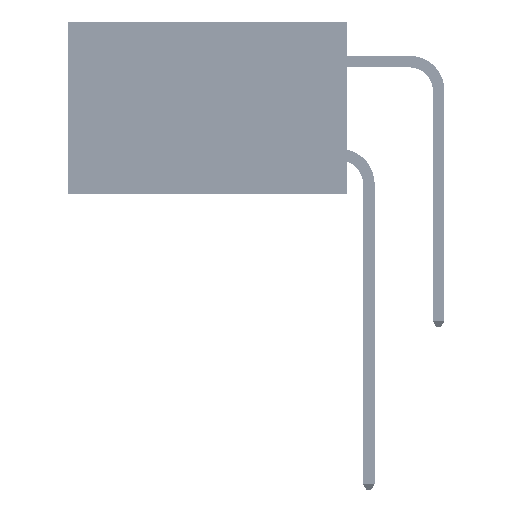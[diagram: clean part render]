
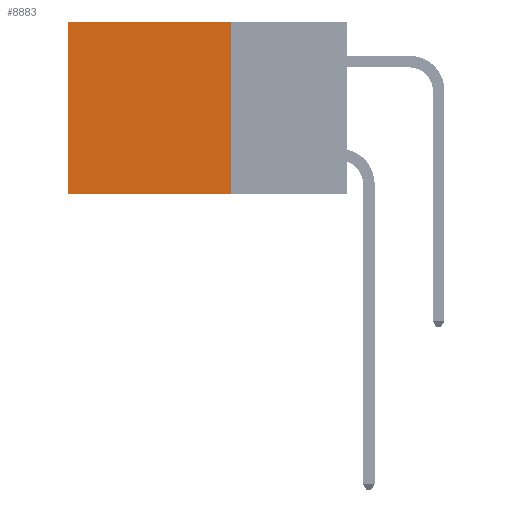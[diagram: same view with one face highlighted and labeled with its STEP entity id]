
A CAD part, left-side view. The second image highlights one B-rep face of the part: STEP entity #8883.
In plain terms, the highlighted planar face has unit normal (-1, 0, 0).
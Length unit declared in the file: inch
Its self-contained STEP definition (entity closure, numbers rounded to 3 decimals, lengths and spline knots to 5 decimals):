
#1233 = CARTESIAN_POINT ( 'NONE',  ( 0.2875, 0.25, 0. ) ) ;
#2089 = CARTESIAN_POINT ( 'NONE',  ( 0.2875, 0.25, -0.37 ) ) ;
#4699 = ORIENTED_EDGE ( 'NONE', *, *, #13519, .F. ) ;
#6615 = LINE ( 'NONE', #29673, #27354 ) ;
#8883 = ADVANCED_FACE ( 'NONE', ( #36243 ), #31109, .F. ) ;
#9104 = DIRECTION ( 'NONE',  ( 0., 1., 0. ) ) ;
#9928 = VERTEX_POINT ( 'NONE', #2089 ) ;
#10130 = VECTOR ( 'NONE', #17261, 39.37008 ) ;
#13519 = EDGE_CURVE ( 'NONE', #16123, #9928, #17411, .T. ) ;
#13660 = CARTESIAN_POINT ( 'NONE',  ( 0.2875, 0.25, 0. ) ) ;
#15400 = ORIENTED_EDGE ( 'NONE', *, *, #16861, .F. ) ;
#16123 = VERTEX_POINT ( 'NONE', #1233 ) ;
#16579 = CARTESIAN_POINT ( 'NONE',  ( 0.2875, 0.25, 0. ) ) ;
#16861 = EDGE_CURVE ( 'NONE', #9928, #22538, #6615, .T. ) ;
#17261 = DIRECTION ( 'NONE',  ( 0., 0., -1. ) ) ;
#17411 = LINE ( 'NONE', #13660, #10130 ) ;
#19578 = LINE ( 'NONE', #30845, #31852 ) ;
#20511 = DIRECTION ( 'NONE',  ( 1., 0., 0. ) ) ;
#20613 = ORIENTED_EDGE ( 'NONE', *, *, #42983, .T. ) ;
#22538 = VERTEX_POINT ( 'NONE', #30517 ) ;
#25399 = EDGE_LOOP ( 'NONE', ( #20613, #15400, #4699, #40472 ) ) ;
#27354 = VECTOR ( 'NONE', #44511, 39.37008 ) ;
#27930 = AXIS2_PLACEMENT_3D ( 'NONE', #16579, #20511, #45489 ) ;
#29030 = CARTESIAN_POINT ( 'NONE',  ( 0.2875, 0.6, 0. ) ) ;
#29673 = CARTESIAN_POINT ( 'NONE',  ( 0.2875, 0.25, -0.37 ) ) ;
#30293 = EDGE_CURVE ( 'NONE', #16123, #36213, #19578, .T. ) ;
#30517 = CARTESIAN_POINT ( 'NONE',  ( 0.2875, 0.6, -0.37 ) ) ;
#30731 = VECTOR ( 'NONE', #32279, 39.37008 ) ;
#30845 = CARTESIAN_POINT ( 'NONE',  ( 0.2875, 0.25, 0. ) ) ;
#31109 = PLANE ( 'NONE',  #27930 ) ;
#31852 = VECTOR ( 'NONE', #9104, 39.37008 ) ;
#32279 = DIRECTION ( 'NONE',  ( 0., 0., -1. ) ) ;
#33496 = LINE ( 'NONE', #44782, #30731 ) ;
#36213 = VERTEX_POINT ( 'NONE', #29030 ) ;
#36243 = FACE_OUTER_BOUND ( 'NONE', #25399, .T. ) ;
#40472 = ORIENTED_EDGE ( 'NONE', *, *, #30293, .T. ) ;
#42983 = EDGE_CURVE ( 'NONE', #36213, #22538, #33496, .T. ) ;
#44511 = DIRECTION ( 'NONE',  ( 0., 1., 0. ) ) ;
#44782 = CARTESIAN_POINT ( 'NONE',  ( 0.2875, 0.6, 0. ) ) ;
#45489 = DIRECTION ( 'NONE',  ( 0., 0., -1. ) ) ;
